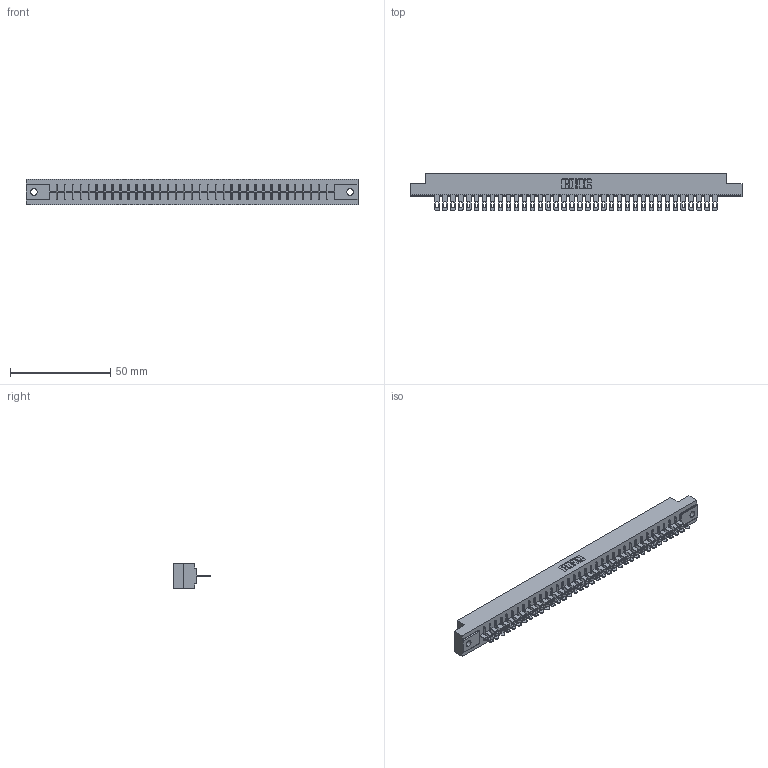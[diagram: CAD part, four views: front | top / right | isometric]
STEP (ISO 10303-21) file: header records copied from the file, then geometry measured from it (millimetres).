
FILE_DESCRIPTION (( 'STEP AP203' ), '1' );
FILE_NAME ('306-036-400-102.STEP', '2020-09-22T04:12:29', ( '' ), ( '' ), 'SwSTEP 2.0', 'SolidWorks 2020', '' );
FILE_SCHEMA (( 'CONFIG_CONTROL_DESIGN' ));
Length unit declared in the file: inch
Products named in the file (3): 306-036-400-102; 306-290-001_100; 306 Part_.128 Dia
Assembly tree (37 placements, depth 2):
  306-036-400-102
    306 Part_.128 Dia
    306-290-001_100  x36
Bounding box: 165.66 x 18.87 x 12.7 mm (x, y, z)
Volume: 18343.1 mm3; surface area: 19123.5 mm2
Topology: 37 solids, 37 shells, 2852 faces, 8056 edges, 5176 vertices
Faces by surface type: plane 1868, cylinder 840, sphere 144
Entity records: 34515 total; most frequent: CARTESIAN_POINT 5795, ORIENTED_EDGE 5744, DIRECTION 5716, EDGE_CURVE 2872, VECTOR 2242, LINE 2242, VERTEX_POINT 1816, AXIS2_PLACEMENT_3D 1737
